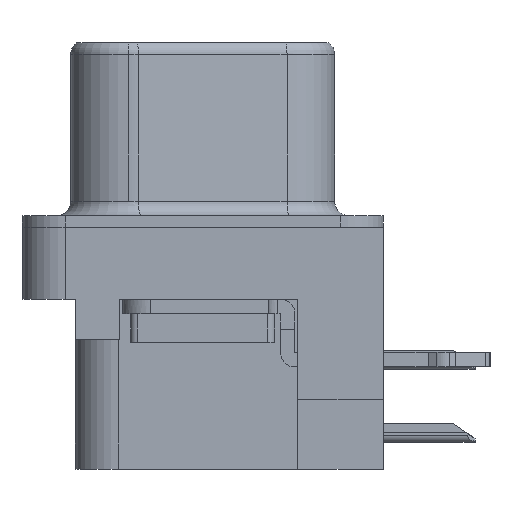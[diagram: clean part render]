
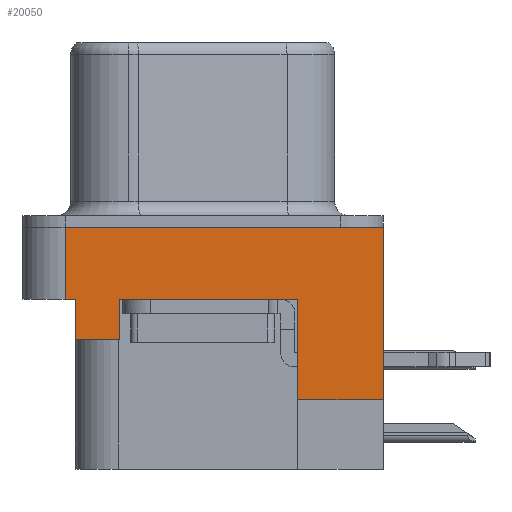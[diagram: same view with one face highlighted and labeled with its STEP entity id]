
A CAD part, left-side view. The second image highlights one B-rep face of the part: STEP entity #20050.
In plain terms, the highlighted planar face has unit normal (-1, 0, 0).
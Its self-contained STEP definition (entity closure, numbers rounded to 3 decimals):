
#107 = ORIENTED_EDGE ( 'NONE', *, *, #691, .T. ) ;
#180 = LINE ( 'NONE', #12463, #12621 ) ;
#252 = CARTESIAN_POINT ( 'NONE',  ( -3., -6.275, -2.5 ) ) ;
#267 = EDGE_CURVE ( 'NONE', #10955, #17820, #13162, .T. ) ;
#377 = CARTESIAN_POINT ( 'NONE',  ( -3., -3.295, -2.5 ) ) ;
#582 = EDGE_CURVE ( 'NONE', #22400, #19515, #8427, .T. ) ;
#618 = FACE_OUTER_BOUND ( 'NONE', #14313, .T. ) ;
#691 = EDGE_CURVE ( 'NONE', #22400, #5522, #10239, .T. ) ;
#827 = EDGE_CURVE ( 'NONE', #20919, #5522, #180, .T. ) ;
#847 = ORIENTED_EDGE ( 'NONE', *, *, #3137, .F. ) ;
#872 = EDGE_CURVE ( 'NONE', #10955, #20919, #20528, .T. ) ;
#970 = EDGE_CURVE ( 'NONE', #19938, #17820, #14455, .T. ) ;
#1015 = EDGE_CURVE ( 'NONE', #19515, #22078, #22403, .T. ) ;
#1180 = ORIENTED_EDGE ( 'NONE', *, *, #582, .F. ) ;
#1914 = ORIENTED_EDGE ( 'NONE', *, *, #15950, .T. ) ;
#2099 = LINE ( 'NONE', #14102, #11467 ) ;
#3009 = ORIENTED_EDGE ( 'NONE', *, *, #18896, .T. ) ;
#3137 = EDGE_CURVE ( 'NONE', #5491, #19938, #2099, .T. ) ;
#3886 = CARTESIAN_POINT ( 'NONE',  ( -3., -6.275, -2.5 ) ) ;
#4088 = CARTESIAN_POINT ( 'NONE',  ( -3., -6.275, -2.5 ) ) ;
#4304 = VECTOR ( 'NONE', #19978, 1000. ) ;
#4370 = CARTESIAN_POINT ( 'NONE',  ( -3., 4.425, -2.5 ) ) ;
#4717 = VECTOR ( 'NONE', #5639, 1000. ) ;
#5480 = DIRECTION ( 'NONE',  ( 0., 0., 1. ) ) ;
#5491 = VERTEX_POINT ( 'NONE', #15713 ) ;
#5522 = VERTEX_POINT ( 'NONE', #14843 ) ;
#5639 = DIRECTION ( 'NONE',  ( 0., 0., 1. ) ) ;
#5697 = DIRECTION ( 'NONE',  ( -1., 0., 0. ) ) ;
#6288 = DIRECTION ( 'NONE',  ( 0., 0., 1. ) ) ;
#6346 = CARTESIAN_POINT ( 'NONE',  ( -3., -6.275, -2.5 ) ) ;
#6451 = VECTOR ( 'NONE', #6288, 1000. ) ;
#6688 = CARTESIAN_POINT ( 'NONE',  ( -3., -6.495, -6. ) ) ;
#6924 = VERTEX_POINT ( 'NONE', #20805 ) ;
#6978 = VECTOR ( 'NONE', #10452, 1000. ) ;
#7455 = PLANE ( 'NONE',  #18365 ) ;
#8427 = LINE ( 'NONE', #6688, #16839 ) ;
#9454 = ORIENTED_EDGE ( 'NONE', *, *, #970, .F. ) ;
#9703 = CARTESIAN_POINT ( 'NONE',  ( -3., 4.775, 0. ) ) ;
#10239 = LINE ( 'NONE', #4088, #14720 ) ;
#10307 = ORIENTED_EDGE ( 'NONE', *, *, #1015, .F. ) ;
#10452 = DIRECTION ( 'NONE',  ( 0., 0., 1. ) ) ;
#10875 = DIRECTION ( 'NONE',  ( 0., -1., 0. ) ) ;
#10955 = VERTEX_POINT ( 'NONE', #18311 ) ;
#11027 = LINE ( 'NONE', #13131, #6451 ) ;
#11126 = DIRECTION ( 'NONE',  ( 0., -1., 0. ) ) ;
#11467 = VECTOR ( 'NONE', #16734, 1000. ) ;
#11953 = ORIENTED_EDGE ( 'NONE', *, *, #872, .F. ) ;
#12463 = CARTESIAN_POINT ( 'NONE',  ( -3., -6.275, 0. ) ) ;
#12621 = VECTOR ( 'NONE', #11126, 1000. ) ;
#13131 = CARTESIAN_POINT ( 'NONE',  ( -3., 2.895, -3.9 ) ) ;
#13162 = LINE ( 'NONE', #252, #17103 ) ;
#14102 = CARTESIAN_POINT ( 'NONE',  ( -3., 4.425, -3.9 ) ) ;
#14226 = CARTESIAN_POINT ( 'NONE',  ( -3., 4.775, -2.5 ) ) ;
#14313 = EDGE_LOOP ( 'NONE', ( #1180, #107, #16030, #11953, #19960, #9454, #847, #3009, #1914, #10307 ) ) ;
#14455 = LINE ( 'NONE', #21379, #4717 ) ;
#14720 = VECTOR ( 'NONE', #16050, 1000. ) ;
#14843 = CARTESIAN_POINT ( 'NONE',  ( -3., -6.275, 0. ) ) ;
#15316 = CARTESIAN_POINT ( 'NONE',  ( -3., -3.295, -8.4 ) ) ;
#15713 = CARTESIAN_POINT ( 'NONE',  ( -3., 2.895, -3.9 ) ) ;
#15950 = EDGE_CURVE ( 'NONE', #6924, #22078, #18578, .T. ) ;
#16030 = ORIENTED_EDGE ( 'NONE', *, *, #827, .F. ) ;
#16050 = DIRECTION ( 'NONE',  ( 0., 0., 1. ) ) ;
#16109 = CARTESIAN_POINT ( 'NONE',  ( -3., -3.295, -6. ) ) ;
#16513 = DIRECTION ( 'NONE',  ( 0., 1., 0. ) ) ;
#16688 = CARTESIAN_POINT ( 'NONE',  ( -3., -6.275, -6. ) ) ;
#16734 = DIRECTION ( 'NONE',  ( 0., 1., 0. ) ) ;
#16839 = VECTOR ( 'NONE', #16513, 1000. ) ;
#17103 = VECTOR ( 'NONE', #10875, 1000. ) ;
#17339 = VECTOR ( 'NONE', #5480, 1000. ) ;
#17667 = DIRECTION ( 'NONE',  ( 0., 0., 1. ) ) ;
#17820 = VERTEX_POINT ( 'NONE', #4370 ) ;
#18311 = CARTESIAN_POINT ( 'NONE',  ( -3., 4.775, -2.5 ) ) ;
#18365 = AXIS2_PLACEMENT_3D ( 'NONE', #3886, #5697, #17667 ) ;
#18578 = LINE ( 'NONE', #6346, #4304 ) ;
#18896 = EDGE_CURVE ( 'NONE', #5491, #6924, #11027, .T. ) ;
#19086 = CARTESIAN_POINT ( 'NONE',  ( -3., 4.425, -3.9 ) ) ;
#19515 = VERTEX_POINT ( 'NONE', #16109 ) ;
#19938 = VERTEX_POINT ( 'NONE', #19086 ) ;
#19960 = ORIENTED_EDGE ( 'NONE', *, *, #267, .T. ) ;
#19978 = DIRECTION ( 'NONE',  ( 0., -1., 0. ) ) ;
#20050 = ADVANCED_FACE ( 'NONE', ( #618 ), #7455, .T. ) ;
#20528 = LINE ( 'NONE', #14226, #6978 ) ;
#20805 = CARTESIAN_POINT ( 'NONE',  ( -3., 2.895, -2.5 ) ) ;
#20919 = VERTEX_POINT ( 'NONE', #9703 ) ;
#21379 = CARTESIAN_POINT ( 'NONE',  ( -3., 4.425, -3.9 ) ) ;
#22078 = VERTEX_POINT ( 'NONE', #377 ) ;
#22400 = VERTEX_POINT ( 'NONE', #16688 ) ;
#22403 = LINE ( 'NONE', #15316, #17339 ) ;
